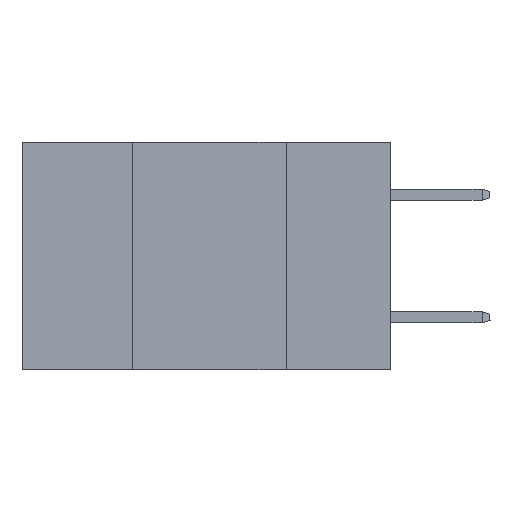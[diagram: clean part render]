
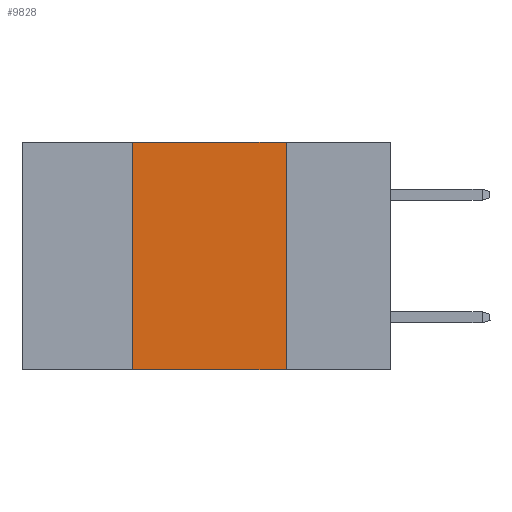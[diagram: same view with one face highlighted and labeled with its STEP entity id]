
A CAD part, left-side view. The second image highlights one B-rep face of the part: STEP entity #9828.
In plain terms, the highlighted planar face has unit normal (-1, 0, 0).
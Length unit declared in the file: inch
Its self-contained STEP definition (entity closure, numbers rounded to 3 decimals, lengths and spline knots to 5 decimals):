
#108 = LINE ( 'NONE', #11371, #3078 ) ;
#1023 = EDGE_CURVE ( 'NONE', #7805, #9440, #2587, .T. ) ;
#1955 = VERTEX_POINT ( 'NONE', #2259 ) ;
#2259 = CARTESIAN_POINT ( 'NONE',  ( 0., 0.17, 0. ) ) ;
#2587 = LINE ( 'NONE', #17777, #4646 ) ;
#2616 = CARTESIAN_POINT ( 'NONE',  ( 0., 0.6, 0. ) ) ;
#3078 = VECTOR ( 'NONE', #14264, 39.37008 ) ;
#3291 = DIRECTION ( 'NONE',  ( 0., -1., 0. ) ) ;
#3914 = CARTESIAN_POINT ( 'NONE',  ( 0., 0.42, -0.37 ) ) ;
#4149 = AXIS2_PLACEMENT_3D ( 'NONE', #2616, #5511, #15228 ) ;
#4646 = VECTOR ( 'NONE', #3291, 39.37008 ) ;
#4737 = CARTESIAN_POINT ( 'NONE',  ( 0., 0.17, -0.37 ) ) ;
#4984 = EDGE_LOOP ( 'NONE', ( #7298, #11423, #6490, #11233 ) ) ;
#5511 = DIRECTION ( 'NONE',  ( 1., 0., 0. ) ) ;
#6192 = DIRECTION ( 'NONE',  ( 0., 0., -1. ) ) ;
#6401 = LINE ( 'NONE', #15905, #13385 ) ;
#6490 = ORIENTED_EDGE ( 'NONE', *, *, #11379, .F. ) ;
#6897 = EDGE_CURVE ( 'NONE', #1955, #9440, #6401, .T. ) ;
#7298 = ORIENTED_EDGE ( 'NONE', *, *, #6897, .F. ) ;
#7805 = VERTEX_POINT ( 'NONE', #3914 ) ;
#8229 = VERTEX_POINT ( 'NONE', #15746 ) ;
#9440 = VERTEX_POINT ( 'NONE', #4737 ) ;
#9828 = ADVANCED_FACE ( 'NONE', ( #11632 ), #13889, .F. ) ;
#11233 = ORIENTED_EDGE ( 'NONE', *, *, #1023, .T. ) ;
#11371 = CARTESIAN_POINT ( 'NONE',  ( 0., 0.42, 0. ) ) ;
#11379 = EDGE_CURVE ( 'NONE', #7805, #8229, #108, .T. ) ;
#11423 = ORIENTED_EDGE ( 'NONE', *, *, #11882, .F. ) ;
#11632 = FACE_OUTER_BOUND ( 'NONE', #4984, .T. ) ;
#11882 = EDGE_CURVE ( 'NONE', #8229, #1955, #12909, .T. ) ;
#12909 = LINE ( 'NONE', #17937, #16134 ) ;
#13385 = VECTOR ( 'NONE', #6192, 39.37008 ) ;
#13889 = PLANE ( 'NONE',  #4149 ) ;
#14264 = DIRECTION ( 'NONE',  ( 0., 0., 1. ) ) ;
#15228 = DIRECTION ( 'NONE',  ( 0., 0., -1. ) ) ;
#15296 = DIRECTION ( 'NONE',  ( 0., -1., 0. ) ) ;
#15746 = CARTESIAN_POINT ( 'NONE',  ( 0., 0.42, 0. ) ) ;
#15905 = CARTESIAN_POINT ( 'NONE',  ( 0., 0.17, 0. ) ) ;
#16134 = VECTOR ( 'NONE', #15296, 39.37008 ) ;
#17777 = CARTESIAN_POINT ( 'NONE',  ( 0., 0.6, -0.37 ) ) ;
#17937 = CARTESIAN_POINT ( 'NONE',  ( 0., 0.6, 0. ) ) ;
